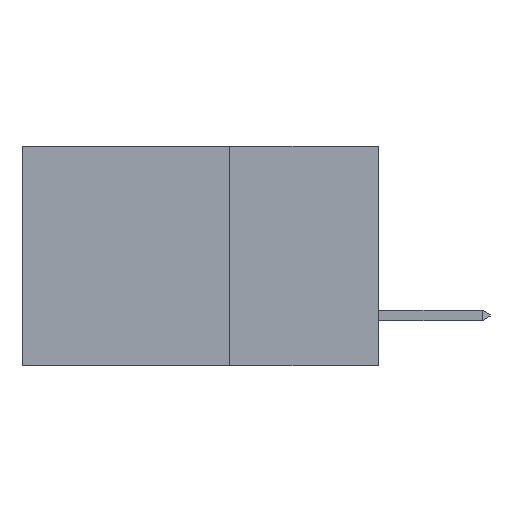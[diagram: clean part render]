
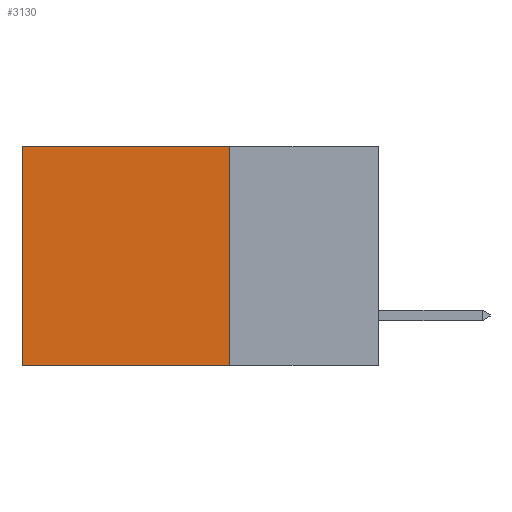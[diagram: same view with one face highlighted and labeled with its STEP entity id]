
A CAD part, left-side view. The second image highlights one B-rep face of the part: STEP entity #3130.
In plain terms, the highlighted planar face has unit normal (-1, 0, 0).
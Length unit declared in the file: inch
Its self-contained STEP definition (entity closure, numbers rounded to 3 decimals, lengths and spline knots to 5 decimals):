
#114 = VERTEX_POINT ( 'NONE', #2013 ) ;
#345 = CARTESIAN_POINT ( 'NONE',  ( 0.2615, 0.25, -0.37 ) ) ;
#561 = VECTOR ( 'NONE', #2234, 39.37008 ) ;
#710 = ORIENTED_EDGE ( 'NONE', *, *, #16732, .F. ) ;
#721 = LINE ( 'NONE', #12593, #10951 ) ;
#958 = EDGE_LOOP ( 'NONE', ( #6668, #710, #5404, #9175 ) ) ;
#1077 = VERTEX_POINT ( 'NONE', #3500 ) ;
#1680 = DIRECTION ( 'NONE',  ( 0., 1., 0. ) ) ;
#1760 = VERTEX_POINT ( 'NONE', #9902 ) ;
#2013 = CARTESIAN_POINT ( 'NONE',  ( 0.2615, 0.25, 0. ) ) ;
#2234 = DIRECTION ( 'NONE',  ( 0., 0., -1. ) ) ;
#3130 = ADVANCED_FACE ( 'NONE', ( #7615 ), #16198, .F. ) ;
#3500 = CARTESIAN_POINT ( 'NONE',  ( 0.2615, 0.6, 0. ) ) ;
#3787 = EDGE_CURVE ( 'NONE', #114, #1760, #721, .T. ) ;
#4641 = LINE ( 'NONE', #345, #7777 ) ;
#5404 = ORIENTED_EDGE ( 'NONE', *, *, #3787, .F. ) ;
#6668 = ORIENTED_EDGE ( 'NONE', *, *, #7765, .T. ) ;
#6950 = CARTESIAN_POINT ( 'NONE',  ( 0.2615, 0.6, -0.37 ) ) ;
#7223 = LINE ( 'NONE', #12399, #561 ) ;
#7615 = FACE_OUTER_BOUND ( 'NONE', #958, .T. ) ;
#7765 = EDGE_CURVE ( 'NONE', #1077, #14866, #7223, .T. ) ;
#7777 = VECTOR ( 'NONE', #1680, 39.37008 ) ;
#8496 = EDGE_CURVE ( 'NONE', #114, #1077, #15867, .T. ) ;
#8824 = VECTOR ( 'NONE', #11242, 39.37008 ) ;
#9175 = ORIENTED_EDGE ( 'NONE', *, *, #8496, .T. ) ;
#9902 = CARTESIAN_POINT ( 'NONE',  ( 0.2615, 0.25, -0.37 ) ) ;
#10951 = VECTOR ( 'NONE', #13486, 39.37008 ) ;
#11242 = DIRECTION ( 'NONE',  ( 0., 1., 0. ) ) ;
#11942 = CARTESIAN_POINT ( 'NONE',  ( 0.2615, 0.25, 0. ) ) ;
#12399 = CARTESIAN_POINT ( 'NONE',  ( 0.2615, 0.6, -0.37 ) ) ;
#12593 = CARTESIAN_POINT ( 'NONE',  ( 0.2615, 0.25, -0.37 ) ) ;
#13180 = AXIS2_PLACEMENT_3D ( 'NONE', #16231, #16177, #16146 ) ;
#13486 = DIRECTION ( 'NONE',  ( 0., 0., -1. ) ) ;
#14866 = VERTEX_POINT ( 'NONE', #6950 ) ;
#15867 = LINE ( 'NONE', #11942, #8824 ) ;
#16146 = DIRECTION ( 'NONE',  ( 0., 0., -1. ) ) ;
#16177 = DIRECTION ( 'NONE',  ( 1., 0., 0. ) ) ;
#16198 = PLANE ( 'NONE',  #13180 ) ;
#16231 = CARTESIAN_POINT ( 'NONE',  ( 0.2615, 0.25, -0.37 ) ) ;
#16732 = EDGE_CURVE ( 'NONE', #1760, #14866, #4641, .T. ) ;
